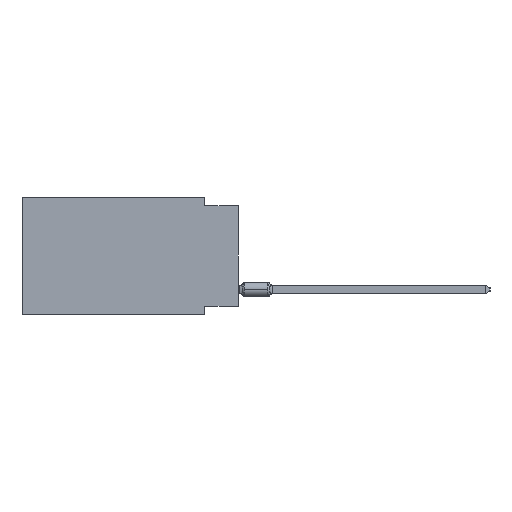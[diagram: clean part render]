
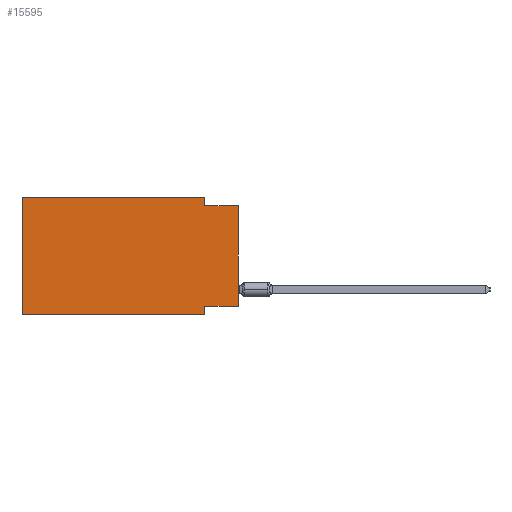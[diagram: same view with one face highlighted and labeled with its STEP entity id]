
A CAD part, left-side view. The second image highlights one B-rep face of the part: STEP entity #15595.
In plain terms, the highlighted planar face has unit normal (-1, 0, 0).
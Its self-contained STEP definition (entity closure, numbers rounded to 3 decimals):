
#931 = DIRECTION ( 'NONE',  ( 0., 1., 0. ) ) ;
#3685 = VECTOR ( 'NONE', #931, 1000. ) ;
#3796 = CARTESIAN_POINT ( 'NONE',  ( 0., 2.54, -8.89 ) ) ;
#3818 = VECTOR ( 'NONE', #16625, 1000. ) ;
#4419 = CARTESIAN_POINT ( 'NONE',  ( 0., 16.383, 0. ) ) ;
#4640 = EDGE_CURVE ( 'NONE', #47999, #24203, #10238, .T. ) ;
#5953 = EDGE_CURVE ( 'NONE', #40299, #47999, #60658, .T. ) ;
#7600 = LINE ( 'NONE', #14380, #27133 ) ;
#8872 = CARTESIAN_POINT ( 'NONE',  ( 0., 16.383, -8.89 ) ) ;
#9302 = CARTESIAN_POINT ( 'NONE',  ( 0., 0., -0.635 ) ) ;
#9336 = CARTESIAN_POINT ( 'NONE',  ( 0., 2.54, -8.89 ) ) ;
#9881 = DIRECTION ( 'NONE',  ( 0., 0., -1. ) ) ;
#10238 = LINE ( 'NONE', #3796, #17228 ) ;
#10417 = CARTESIAN_POINT ( 'NONE',  ( 0., 0., -0.635 ) ) ;
#12521 = ORIENTED_EDGE ( 'NONE', *, *, #66989, .T. ) ;
#12987 = EDGE_CURVE ( 'NONE', #39973, #50525, #23741, .T. ) ;
#13677 = ORIENTED_EDGE ( 'NONE', *, *, #62207, .F. ) ;
#14380 = CARTESIAN_POINT ( 'NONE',  ( 0., 16.383, 0. ) ) ;
#14579 = CARTESIAN_POINT ( 'NONE',  ( 0., 0., 0. ) ) ;
#15196 = CARTESIAN_POINT ( 'NONE',  ( 0., 2.54, 0. ) ) ;
#15595 = ADVANCED_FACE ( 'NONE', ( #40639 ), #19532, .F. ) ;
#15687 = EDGE_CURVE ( 'NONE', #62189, #39973, #48822, .T. ) ;
#16625 = DIRECTION ( 'NONE',  ( 0., 0., -1. ) ) ;
#17228 = VECTOR ( 'NONE', #9881, 1000. ) ;
#17296 = EDGE_LOOP ( 'NONE', ( #56102, #69542, #35841, #28194, #13677, #12521, #62907, #46768 ) ) ;
#18008 = CARTESIAN_POINT ( 'NONE',  ( 0., 0., -8.255 ) ) ;
#18822 = DIRECTION ( 'NONE',  ( 1., 0., 0. ) ) ;
#19532 = PLANE ( 'NONE',  #50656 ) ;
#23741 = LINE ( 'NONE', #9302, #65221 ) ;
#23743 = VECTOR ( 'NONE', #42012, 1000. ) ;
#24064 = DIRECTION ( 'NONE',  ( 0., -1., 0. ) ) ;
#24203 = VERTEX_POINT ( 'NONE', #9336 ) ;
#24662 = VERTEX_POINT ( 'NONE', #51851 ) ;
#24978 = LINE ( 'NONE', #14579, #61837 ) ;
#25069 = DIRECTION ( 'NONE',  ( 0., -1., 0. ) ) ;
#25948 = DIRECTION ( 'NONE',  ( 0., 0., -1. ) ) ;
#27133 = VECTOR ( 'NONE', #24064, 1000. ) ;
#28194 = ORIENTED_EDGE ( 'NONE', *, *, #61368, .F. ) ;
#29643 = CARTESIAN_POINT ( 'NONE',  ( 0., 2.54, 0. ) ) ;
#29991 = LINE ( 'NONE', #62507, #23743 ) ;
#31319 = CARTESIAN_POINT ( 'NONE',  ( 0., 16.383, 0. ) ) ;
#35841 = ORIENTED_EDGE ( 'NONE', *, *, #15687, .F. ) ;
#36418 = DIRECTION ( 'NONE',  ( 0., 0., 1. ) ) ;
#37124 = LINE ( 'NONE', #8872, #49262 ) ;
#37508 = CARTESIAN_POINT ( 'NONE',  ( 0., 2.54, -8.255 ) ) ;
#38870 = CARTESIAN_POINT ( 'NONE',  ( 0., 0., -8.255 ) ) ;
#39973 = VERTEX_POINT ( 'NONE', #47387 ) ;
#40299 = VERTEX_POINT ( 'NONE', #18008 ) ;
#40639 = FACE_OUTER_BOUND ( 'NONE', #17296, .T. ) ;
#42012 = DIRECTION ( 'NONE',  ( 0., 0., 1. ) ) ;
#42829 = DIRECTION ( 'NONE',  ( 0., -1., 0. ) ) ;
#46768 = ORIENTED_EDGE ( 'NONE', *, *, #5953, .F. ) ;
#47387 = CARTESIAN_POINT ( 'NONE',  ( 0., 2.54, -0.635 ) ) ;
#47999 = VERTEX_POINT ( 'NONE', #37508 ) ;
#48822 = LINE ( 'NONE', #15196, #3818 ) ;
#49262 = VECTOR ( 'NONE', #42829, 1000. ) ;
#50525 = VERTEX_POINT ( 'NONE', #10417 ) ;
#50656 = AXIS2_PLACEMENT_3D ( 'NONE', #31319, #18822, #25948 ) ;
#51356 = EDGE_CURVE ( 'NONE', #40299, #50525, #24978, .T. ) ;
#51851 = CARTESIAN_POINT ( 'NONE',  ( 0., 16.383, -8.89 ) ) ;
#56102 = ORIENTED_EDGE ( 'NONE', *, *, #51356, .T. ) ;
#59818 = VERTEX_POINT ( 'NONE', #4419 ) ;
#60658 = LINE ( 'NONE', #38870, #3685 ) ;
#61368 = EDGE_CURVE ( 'NONE', #59818, #62189, #7600, .T. ) ;
#61837 = VECTOR ( 'NONE', #36418, 1000. ) ;
#62189 = VERTEX_POINT ( 'NONE', #29643 ) ;
#62207 = EDGE_CURVE ( 'NONE', #24662, #59818, #29991, .T. ) ;
#62507 = CARTESIAN_POINT ( 'NONE',  ( 0., 16.383, 0. ) ) ;
#62907 = ORIENTED_EDGE ( 'NONE', *, *, #4640, .F. ) ;
#65221 = VECTOR ( 'NONE', #25069, 1000. ) ;
#66989 = EDGE_CURVE ( 'NONE', #24662, #24203, #37124, .T. ) ;
#69542 = ORIENTED_EDGE ( 'NONE', *, *, #12987, .F. ) ;
